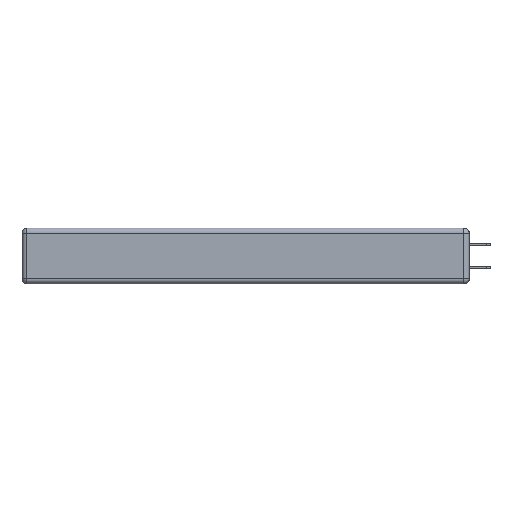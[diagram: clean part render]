
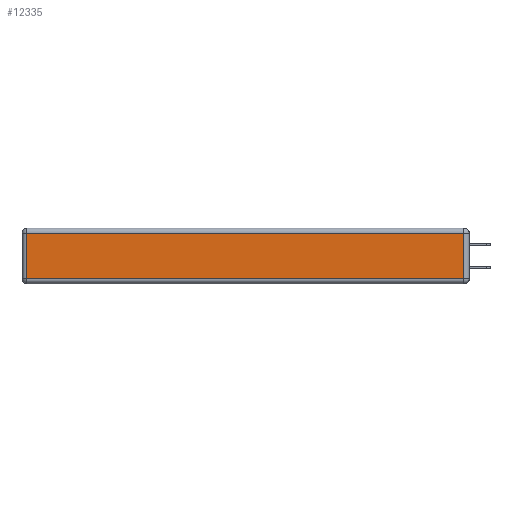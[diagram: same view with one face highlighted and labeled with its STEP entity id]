
A CAD part, left-side view. The second image highlights one B-rep face of the part: STEP entity #12335.
In plain terms, the highlighted planar face has unit normal (-1, 0, 0).
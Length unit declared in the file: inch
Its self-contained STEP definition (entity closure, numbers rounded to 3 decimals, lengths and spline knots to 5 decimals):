
#251 = VERTEX_POINT ( 'NONE', #12847 ) ;
#294 = ORIENTED_EDGE ( 'NONE', *, *, #16836, .T. ) ;
#1277 = EDGE_CURVE ( 'NONE', #8838, #251, #5264, .T. ) ;
#1803 = AXIS2_PLACEMENT_3D ( 'NONE', #13048, #15744, #10498 ) ;
#1907 = CARTESIAN_POINT ( 'NONE',  ( 0., 0., -0.313 ) ) ;
#4038 = CARTESIAN_POINT ( 'NONE',  ( 0., 2.72, -0.313 ) ) ;
#4843 = VECTOR ( 'NONE', #16690, 39.37008 ) ;
#5212 = LINE ( 'NONE', #14300, #9812 ) ;
#5264 = LINE ( 'NONE', #1907, #4843 ) ;
#8838 = VERTEX_POINT ( 'NONE', #4038 ) ;
#9112 = VECTOR ( 'NONE', #9494, 39.37008 ) ;
#9494 = DIRECTION ( 'NONE',  ( 0., 1., 0. ) ) ;
#9812 = VECTOR ( 'NONE', #17037, 39.37008 ) ;
#10022 = DIRECTION ( 'NONE',  ( 0., 0., -1. ) ) ;
#10498 = DIRECTION ( 'NONE',  ( 0., 0., 1. ) ) ;
#10702 = ORIENTED_EDGE ( 'NONE', *, *, #12811, .T. ) ;
#11004 = CARTESIAN_POINT ( 'NONE',  ( 0., 0.03, -0.03 ) ) ;
#11018 = EDGE_CURVE ( 'NONE', #251, #15596, #5212, .T. ) ;
#12136 = CARTESIAN_POINT ( 'NONE',  ( 0., 2.75, -0.03 ) ) ;
#12335 = ADVANCED_FACE ( 'NONE', ( #17129 ), #15683, .T. ) ;
#12624 = CARTESIAN_POINT ( 'NONE',  ( 0., 2.72, -0.343 ) ) ;
#12680 = LINE ( 'NONE', #12136, #9112 ) ;
#12722 = VECTOR ( 'NONE', #10022, 39.37008 ) ;
#12811 = EDGE_CURVE ( 'NONE', #13344, #8838, #16909, .T. ) ;
#12847 = CARTESIAN_POINT ( 'NONE',  ( 0., 0.03, -0.313 ) ) ;
#13048 = CARTESIAN_POINT ( 'NONE',  ( 0., 0., -0.343 ) ) ;
#13344 = VERTEX_POINT ( 'NONE', #15245 ) ;
#14300 = CARTESIAN_POINT ( 'NONE',  ( 0., 0.03, -0.343 ) ) ;
#15236 = EDGE_LOOP ( 'NONE', ( #16881, #15730, #294, #10702 ) ) ;
#15245 = CARTESIAN_POINT ( 'NONE',  ( 0., 2.72, -0.03 ) ) ;
#15596 = VERTEX_POINT ( 'NONE', #11004 ) ;
#15683 = PLANE ( 'NONE',  #1803 ) ;
#15730 = ORIENTED_EDGE ( 'NONE', *, *, #11018, .T. ) ;
#15744 = DIRECTION ( 'NONE',  ( -1., 0., 0. ) ) ;
#16690 = DIRECTION ( 'NONE',  ( 0., -1., 0. ) ) ;
#16836 = EDGE_CURVE ( 'NONE', #15596, #13344, #12680, .T. ) ;
#16881 = ORIENTED_EDGE ( 'NONE', *, *, #1277, .T. ) ;
#16909 = LINE ( 'NONE', #12624, #12722 ) ;
#17037 = DIRECTION ( 'NONE',  ( 0., 0., 1. ) ) ;
#17129 = FACE_OUTER_BOUND ( 'NONE', #15236, .T. ) ;
